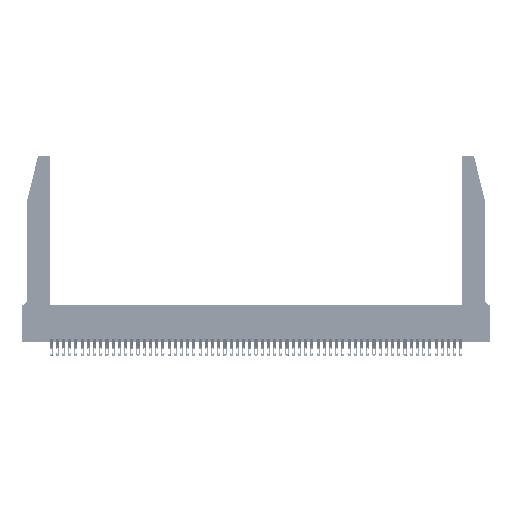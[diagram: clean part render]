
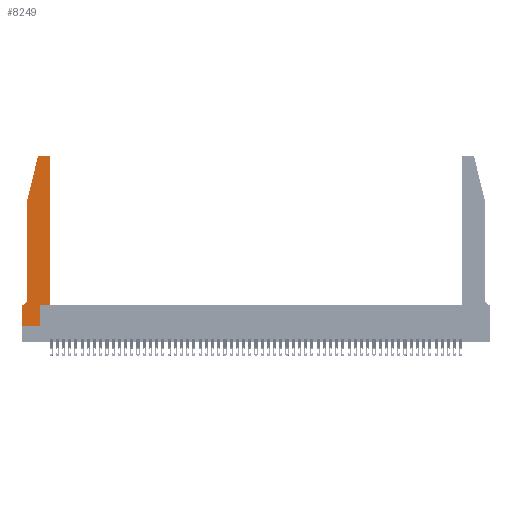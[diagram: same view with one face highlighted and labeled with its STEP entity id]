
A CAD part, top view. The second image highlights one B-rep face of the part: STEP entity #8249.
In plain terms, the highlighted planar face has unit normal (0, 0, 1).
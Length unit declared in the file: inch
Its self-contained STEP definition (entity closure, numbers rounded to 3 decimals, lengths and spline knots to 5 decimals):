
#23 = DIRECTION ( 'NONE',  ( -1., 0., 0. ) ) ;
#2055 = CARTESIAN_POINT ( 'NONE',  ( 0.0755, 2., 0.37 ) ) ;
#2231 = VERTEX_POINT ( 'NONE', #23896 ) ;
#3746 = PLANE ( 'NONE',  #6304 ) ;
#5149 = VERTEX_POINT ( 'NONE', #44117 ) ;
#5301 = LINE ( 'NONE', #13821, #6619 ) ;
#6304 = AXIS2_PLACEMENT_3D ( 'NONE', #41188, #49752, #24088 ) ;
#6619 = VECTOR ( 'NONE', #30516, 39.37008 ) ;
#8120 = CARTESIAN_POINT ( 'NONE',  ( 0.4205, 2.72, 0.37 ) ) ;
#8217 = VECTOR ( 'NONE', #23128, 39.37008 ) ;
#8249 = ADVANCED_FACE ( 'NONE', ( #37301 ), #3746, .T. ) ;
#8662 = CARTESIAN_POINT ( 'NONE',  ( 0.0755, 2., 0.37 ) ) ;
#8998 = ORIENTED_EDGE ( 'NONE', *, *, #53187, .T. ) ;
#9252 = CARTESIAN_POINT ( 'NONE',  ( 0.4505, 0.35, 0.37 ) ) ;
#10606 = ORIENTED_EDGE ( 'NONE', *, *, #29997, .T. ) ;
#10636 = VERTEX_POINT ( 'NONE', #48797 ) ;
#10794 = LINE ( 'NONE', #49482, #19963 ) ;
#13064 = DIRECTION ( 'NONE',  ( -0.239, -0.971, 0. ) ) ;
#13821 = CARTESIAN_POINT ( 'NONE',  ( 0.2865, 0.35, 0.37 ) ) ;
#13825 = ORIENTED_EDGE ( 'NONE', *, *, #15366, .T. ) ;
#14103 = ORIENTED_EDGE ( 'NONE', *, *, #51812, .T. ) ;
#14721 = LINE ( 'NONE', #31027, #8217 ) ;
#15153 = EDGE_LOOP ( 'NONE', ( #13825, #43725, #45510, #10606, #33857, #23990, #46061, #8998, #42027, #29108, #14103, #22999 ) ) ;
#15366 = EDGE_CURVE ( 'NONE', #32937, #41514, #43235, .T. ) ;
#16528 = VECTOR ( 'NONE', #23, 39.37008 ) ;
#16713 = VECTOR ( 'NONE', #38967, 39.37008 ) ;
#17201 = AXIS2_PLACEMENT_3D ( 'NONE', #46832, #51207, #52466 ) ;
#17916 = EDGE_CURVE ( 'NONE', #43626, #28756, #5301, .T. ) ;
#19963 = VECTOR ( 'NONE', #24373, 39.37008 ) ;
#20505 = EDGE_CURVE ( 'NONE', #5149, #40613, #20707, .T. ) ;
#20707 = CIRCLE ( 'NONE', #17201, 0.07 ) ;
#20884 = VERTEX_POINT ( 'NONE', #27167 ) ;
#21200 = EDGE_CURVE ( 'NONE', #52385, #22796, #10794, .T. ) ;
#21477 = CARTESIAN_POINT ( 'NONE',  ( 0.0755, 2., 0.37 ) ) ;
#22796 = VERTEX_POINT ( 'NONE', #47874 ) ;
#22999 = ORIENTED_EDGE ( 'NONE', *, *, #50413, .T. ) ;
#23128 = DIRECTION ( 'NONE',  ( 1., 0., 0. ) ) ;
#23615 = CARTESIAN_POINT ( 'NONE',  ( 0.2865, 0., 0.37 ) ) ;
#23896 = CARTESIAN_POINT ( 'NONE',  ( 0.25487, 2.72718, 0.37 ) ) ;
#23990 = ORIENTED_EDGE ( 'NONE', *, *, #38194, .T. ) ;
#24088 = DIRECTION ( 'NONE',  ( 1., 0., 0. ) ) ;
#24373 = DIRECTION ( 'NONE',  ( 0., -1., 0. ) ) ;
#25045 = DIRECTION ( 'NONE',  ( 0., 0., 1. ) ) ;
#25177 = VERTEX_POINT ( 'NONE', #21477 ) ;
#27167 = CARTESIAN_POINT ( 'NONE',  ( 0.4505, 0.35, 0.37 ) ) ;
#27895 = EDGE_CURVE ( 'NONE', #2231, #25177, #54002, .T. ) ;
#28756 = VERTEX_POINT ( 'NONE', #49639 ) ;
#28791 = AXIS2_PLACEMENT_3D ( 'NONE', #8120, #45703, #49914 ) ;
#29108 = ORIENTED_EDGE ( 'NONE', *, *, #32326, .T. ) ;
#29230 = LINE ( 'NONE', #2055, #16713 ) ;
#29997 = EDGE_CURVE ( 'NONE', #25177, #5149, #29230, .T. ) ;
#30516 = DIRECTION ( 'NONE',  ( 0., 1., 0. ) ) ;
#30981 = VECTOR ( 'NONE', #47006, 39.37008 ) ;
#31027 = CARTESIAN_POINT ( 'NONE',  ( 0., 0., 0.37 ) ) ;
#31272 = CARTESIAN_POINT ( 'NONE',  ( 0., 0.35, 0.37 ) ) ;
#32319 = LINE ( 'NONE', #9252, #30981 ) ;
#32326 = EDGE_CURVE ( 'NONE', #28756, #20884, #32319, .T. ) ;
#32937 = VERTEX_POINT ( 'NONE', #39891 ) ;
#33146 = CARTESIAN_POINT ( 'NONE',  ( 0.284, 2.72, 0.37 ) ) ;
#33857 = ORIENTED_EDGE ( 'NONE', *, *, #20505, .T. ) ;
#35039 = CARTESIAN_POINT ( 'NONE',  ( 0.4505, 0.35, 0.37 ) ) ;
#36603 = VECTOR ( 'NONE', #51841, 39.37008 ) ;
#37301 = FACE_OUTER_BOUND ( 'NONE', #15153, .T. ) ;
#38194 = EDGE_CURVE ( 'NONE', #40613, #52385, #53919, .T. ) ;
#38967 = DIRECTION ( 'NONE',  ( 0., -1., 0. ) ) ;
#39891 = CARTESIAN_POINT ( 'NONE',  ( 0.4205, 2.75, 0.37 ) ) ;
#40613 = VERTEX_POINT ( 'NONE', #52309 ) ;
#41188 = CARTESIAN_POINT ( 'NONE',  ( 0., 0.35, 0.37 ) ) ;
#41514 = VERTEX_POINT ( 'NONE', #46560 ) ;
#41614 = VECTOR ( 'NONE', #13064, 39.37008 ) ;
#41909 = CIRCLE ( 'NONE', #28791, 0.03 ) ;
#42027 = ORIENTED_EDGE ( 'NONE', *, *, #17916, .T. ) ;
#42707 = AXIS2_PLACEMENT_3D ( 'NONE', #33146, #25045, #53988 ) ;
#42976 = CIRCLE ( 'NONE', #42707, 0.03 ) ;
#43235 = LINE ( 'NONE', #53930, #47155 ) ;
#43626 = VERTEX_POINT ( 'NONE', #23615 ) ;
#43725 = ORIENTED_EDGE ( 'NONE', *, *, #45467, .T. ) ;
#44117 = CARTESIAN_POINT ( 'NONE',  ( 0.0755, 0.42, 0.37 ) ) ;
#45467 = EDGE_CURVE ( 'NONE', #41514, #2231, #42976, .T. ) ;
#45510 = ORIENTED_EDGE ( 'NONE', *, *, #27895, .T. ) ;
#45703 = DIRECTION ( 'NONE',  ( 0., 0., 1. ) ) ;
#46061 = ORIENTED_EDGE ( 'NONE', *, *, #21200, .T. ) ;
#46439 = CARTESIAN_POINT ( 'NONE',  ( 0.0755, 0.35, 0.37 ) ) ;
#46560 = CARTESIAN_POINT ( 'NONE',  ( 0.284, 2.75, 0.37 ) ) ;
#46832 = CARTESIAN_POINT ( 'NONE',  ( 0.0055, 0.42, 0.37 ) ) ;
#47006 = DIRECTION ( 'NONE',  ( 1., 0., 0. ) ) ;
#47155 = VECTOR ( 'NONE', #54110, 39.37008 ) ;
#47705 = LINE ( 'NONE', #35039, #36603 ) ;
#47874 = CARTESIAN_POINT ( 'NONE',  ( 0., 0., 0.37 ) ) ;
#48797 = CARTESIAN_POINT ( 'NONE',  ( 0.4505, 2.72, 0.37 ) ) ;
#49482 = CARTESIAN_POINT ( 'NONE',  ( 0., 0., 0.37 ) ) ;
#49639 = CARTESIAN_POINT ( 'NONE',  ( 0.2865, 0.35, 0.37 ) ) ;
#49752 = DIRECTION ( 'NONE',  ( 0., 0., 1. ) ) ;
#49914 = DIRECTION ( 'NONE',  ( 1., 0., 0. ) ) ;
#50413 = EDGE_CURVE ( 'NONE', #10636, #32937, #41909, .T. ) ;
#51207 = DIRECTION ( 'NONE',  ( 0., 0., -1. ) ) ;
#51812 = EDGE_CURVE ( 'NONE', #20884, #10636, #47705, .T. ) ;
#51841 = DIRECTION ( 'NONE',  ( 0., 1., 0. ) ) ;
#52309 = CARTESIAN_POINT ( 'NONE',  ( 0.0055, 0.35, 0.37 ) ) ;
#52385 = VERTEX_POINT ( 'NONE', #31272 ) ;
#52466 = DIRECTION ( 'NONE',  ( -1., 0., 0. ) ) ;
#53187 = EDGE_CURVE ( 'NONE', #22796, #43626, #14721, .T. ) ;
#53919 = LINE ( 'NONE', #46439, #16528 ) ;
#53930 = CARTESIAN_POINT ( 'NONE',  ( 0.2605, 2.75, 0.37 ) ) ;
#53988 = DIRECTION ( 'NONE',  ( 1., 0., 0. ) ) ;
#54002 = LINE ( 'NONE', #8662, #41614 ) ;
#54110 = DIRECTION ( 'NONE',  ( -1., 0., 0. ) ) ;
